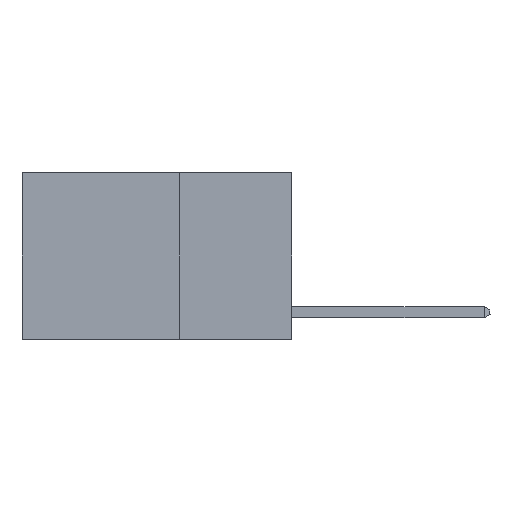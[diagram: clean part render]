
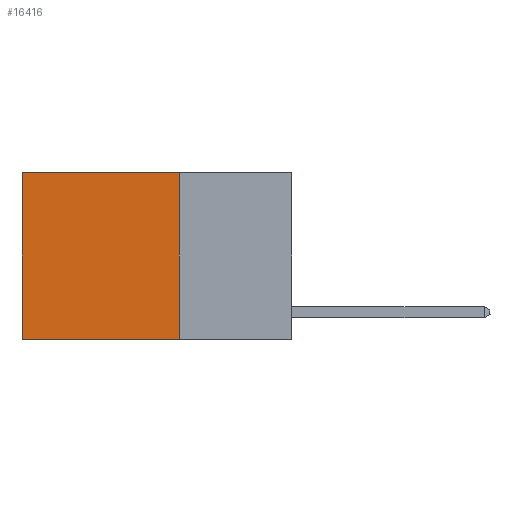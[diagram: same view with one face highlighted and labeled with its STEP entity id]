
A CAD part, left-side view. The second image highlights one B-rep face of the part: STEP entity #16416.
In plain terms, the highlighted planar face has unit normal (-1, 0, 0).
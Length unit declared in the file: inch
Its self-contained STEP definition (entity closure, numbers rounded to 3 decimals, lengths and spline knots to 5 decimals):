
#858 = ORIENTED_EDGE ( 'NONE', *, *, #9432, .F. ) ;
#4944 = EDGE_CURVE ( 'NONE', #14996, #8570, #17820, .T. ) ;
#4952 = VECTOR ( 'NONE', #26166, 39.37008 ) ;
#5997 = EDGE_LOOP ( 'NONE', ( #28175, #13876, #858, #7346 ) ) ;
#6017 = CARTESIAN_POINT ( 'NONE',  ( 0.2625, 0.25, -0.37 ) ) ;
#6259 = CARTESIAN_POINT ( 'NONE',  ( 0.2625, 0.6, 0. ) ) ;
#6326 = FACE_OUTER_BOUND ( 'NONE', #5997, .T. ) ;
#7187 = CARTESIAN_POINT ( 'NONE',  ( 0.2625, 0.25, -0.37 ) ) ;
#7346 = ORIENTED_EDGE ( 'NONE', *, *, #17882, .T. ) ;
#8249 = LINE ( 'NONE', #6017, #23849 ) ;
#8353 = CARTESIAN_POINT ( 'NONE',  ( 0.2625, 0.6, 0. ) ) ;
#8481 = DIRECTION ( 'NONE',  ( 0., 0., -1. ) ) ;
#8570 = VERTEX_POINT ( 'NONE', #29093 ) ;
#9432 = EDGE_CURVE ( 'NONE', #26133, #20277, #13944, .T. ) ;
#11418 = CARTESIAN_POINT ( 'NONE',  ( 0.2625, 0.25, 0. ) ) ;
#11719 = DIRECTION ( 'NONE',  ( 0., 0., -1. ) ) ;
#12326 = VECTOR ( 'NONE', #8481, 39.37008 ) ;
#13876 = ORIENTED_EDGE ( 'NONE', *, *, #14567, .F. ) ;
#13944 = LINE ( 'NONE', #23112, #17293 ) ;
#14567 = EDGE_CURVE ( 'NONE', #20277, #8570, #8249, .T. ) ;
#14996 = VERTEX_POINT ( 'NONE', #8353 ) ;
#15079 = DIRECTION ( 'NONE',  ( 0., 1., 0. ) ) ;
#15384 = PLANE ( 'NONE',  #17270 ) ;
#16416 = ADVANCED_FACE ( 'NONE', ( #6326 ), #15384, .F. ) ;
#17270 = AXIS2_PLACEMENT_3D ( 'NONE', #24412, #22186, #28974 ) ;
#17293 = VECTOR ( 'NONE', #11719, 39.37008 ) ;
#17820 = LINE ( 'NONE', #6259, #12326 ) ;
#17882 = EDGE_CURVE ( 'NONE', #26133, #14996, #19220, .T. ) ;
#19220 = LINE ( 'NONE', #21581, #4952 ) ;
#20277 = VERTEX_POINT ( 'NONE', #7187 ) ;
#21581 = CARTESIAN_POINT ( 'NONE',  ( 0.2625, 0.25, 0. ) ) ;
#22186 = DIRECTION ( 'NONE',  ( 1., 0., 0. ) ) ;
#23112 = CARTESIAN_POINT ( 'NONE',  ( 0.2625, 0.25, 0. ) ) ;
#23849 = VECTOR ( 'NONE', #15079, 39.37008 ) ;
#24412 = CARTESIAN_POINT ( 'NONE',  ( 0.2625, 0.25, 0. ) ) ;
#26133 = VERTEX_POINT ( 'NONE', #11418 ) ;
#26166 = DIRECTION ( 'NONE',  ( 0., 1., 0. ) ) ;
#28175 = ORIENTED_EDGE ( 'NONE', *, *, #4944, .T. ) ;
#28974 = DIRECTION ( 'NONE',  ( 0., 0., -1. ) ) ;
#29093 = CARTESIAN_POINT ( 'NONE',  ( 0.2625, 0.6, -0.37 ) ) ;
